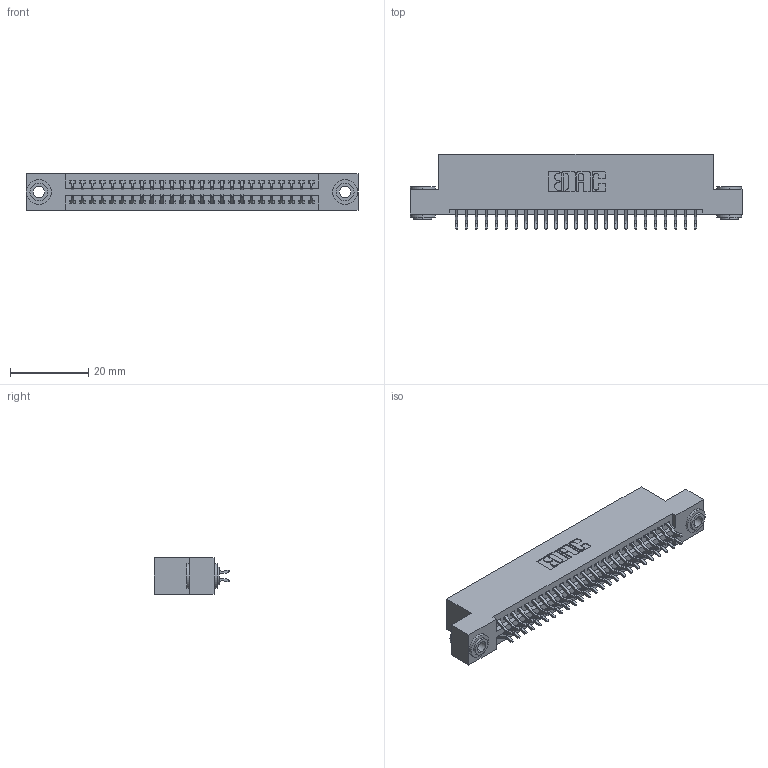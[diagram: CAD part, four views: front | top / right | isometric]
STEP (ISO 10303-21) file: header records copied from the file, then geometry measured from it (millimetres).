
FILE_DESCRIPTION (( 'STEP AP203' ), '1' );
FILE_NAME ('395-050-556-203.STEP', '2018-11-20T10:01:33', ( '' ), ( '' ), 'SwSTEP 2.0', 'SolidWorks 2016', '' );
FILE_SCHEMA (( 'CONFIG_CONTROL_DESIGN' ));
Length unit declared in the file: inch
Products named in the file (4): 345-250-002_345-250-002-102; 345 Part_Flush Mounting Lugs - 0.156 Dia-TH; 395-050-556-203; 345-292-001_556 Tail
Assembly tree (53 placements, depth 2):
  395-050-556-203
    345 Part_Flush Mounting Lugs - 0.156 Dia-TH
    345-292-001_556 Tail  x50
    345-250-002_345-250-002-102  x2
Bounding box: 84.71 x 19.24 x 9.4 mm (x, y, z)
Volume: 8088.3 mm3; surface area: 11787.8 mm2
Topology: 53 solids, 53 shells, 2964 faces, 8767 edges, 5774 vertices
Faces by surface type: plane 1940, cylinder 1016, cone 8
Entity records: 22774 total; most frequent: CARTESIAN_POINT 3823, ORIENTED_EDGE 3738, DIRECTION 3411, EDGE_CURVE 1869, LINE 1605, VECTOR 1605, VERTEX_POINT 1242, AXIS2_PLACEMENT_3D 903
